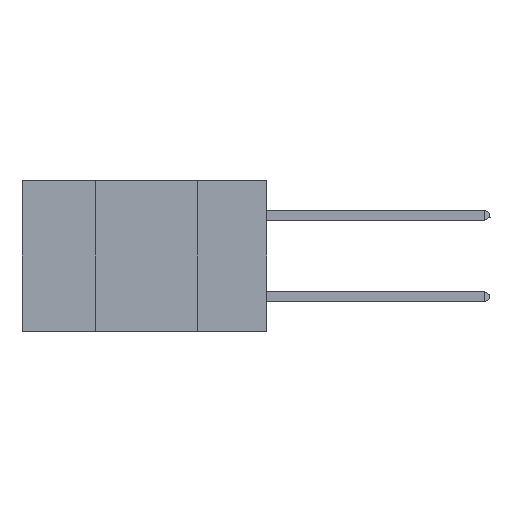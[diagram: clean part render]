
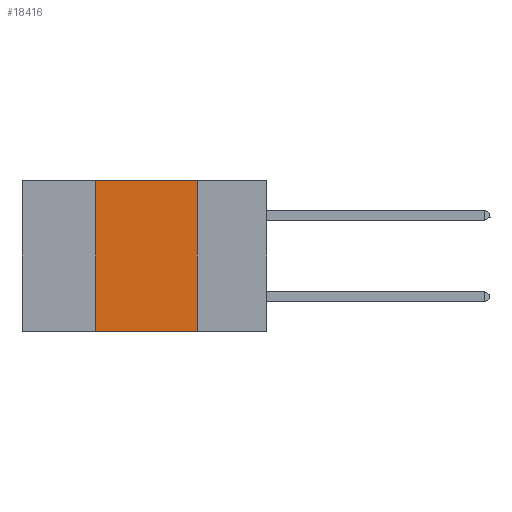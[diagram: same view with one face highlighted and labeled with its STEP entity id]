
A CAD part, left-side view. The second image highlights one B-rep face of the part: STEP entity #18416.
In plain terms, the highlighted planar face has unit normal (-1, 0, 0).
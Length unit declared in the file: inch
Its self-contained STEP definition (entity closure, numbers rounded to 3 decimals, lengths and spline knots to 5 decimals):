
#700 = CARTESIAN_POINT ( 'NONE',  ( 0., 0.42, -0.37 ) ) ;
#1457 = ORIENTED_EDGE ( 'NONE', *, *, #24582, .F. ) ;
#3291 = VERTEX_POINT ( 'NONE', #20561 ) ;
#4500 = LINE ( 'NONE', #32602, #20239 ) ;
#4933 = ORIENTED_EDGE ( 'NONE', *, *, #39990, .F. ) ;
#5363 = EDGE_CURVE ( 'NONE', #10061, #11072, #24682, .T. ) ;
#6220 = ORIENTED_EDGE ( 'NONE', *, *, #5363, .F. ) ;
#8501 = FACE_OUTER_BOUND ( 'NONE', #34142, .T. ) ;
#8634 = DIRECTION ( 'NONE',  ( 0., -1., 0. ) ) ;
#10061 = VERTEX_POINT ( 'NONE', #700 ) ;
#10278 = DIRECTION ( 'NONE',  ( 0., 0., 1. ) ) ;
#11072 = VERTEX_POINT ( 'NONE', #42712 ) ;
#11085 = PLANE ( 'NONE',  #21429 ) ;
#12824 = VECTOR ( 'NONE', #10278, 39.37008 ) ;
#15388 = LINE ( 'NONE', #29550, #35686 ) ;
#18416 = ADVANCED_FACE ( 'NONE', ( #8501 ), #11085, .F. ) ;
#20239 = VECTOR ( 'NONE', #45882, 39.37008 ) ;
#20561 = CARTESIAN_POINT ( 'NONE',  ( 0., 0.17, -0.37 ) ) ;
#21429 = AXIS2_PLACEMENT_3D ( 'NONE', #29192, #39649, #32898 ) ;
#21644 = CARTESIAN_POINT ( 'NONE',  ( 0., 0.42, 0. ) ) ;
#24582 = EDGE_CURVE ( 'NONE', #40576, #3291, #4500, .T. ) ;
#24682 = LINE ( 'NONE', #21644, #12824 ) ;
#25158 = DIRECTION ( 'NONE',  ( 0., -1., 0. ) ) ;
#29192 = CARTESIAN_POINT ( 'NONE',  ( 0., 0.6, 0. ) ) ;
#29242 = VECTOR ( 'NONE', #8634, 39.37008 ) ;
#29550 = CARTESIAN_POINT ( 'NONE',  ( 0., 0.6, -0.37 ) ) ;
#32602 = CARTESIAN_POINT ( 'NONE',  ( 0., 0.17, 0. ) ) ;
#32898 = DIRECTION ( 'NONE',  ( 0., 0., -1. ) ) ;
#33898 = CARTESIAN_POINT ( 'NONE',  ( 0., 0.17, 0. ) ) ;
#34142 = EDGE_LOOP ( 'NONE', ( #1457, #4933, #6220, #39205 ) ) ;
#35686 = VECTOR ( 'NONE', #25158, 39.37008 ) ;
#36899 = EDGE_CURVE ( 'NONE', #10061, #3291, #15388, .T. ) ;
#39205 = ORIENTED_EDGE ( 'NONE', *, *, #36899, .T. ) ;
#39649 = DIRECTION ( 'NONE',  ( 1., 0., 0. ) ) ;
#39990 = EDGE_CURVE ( 'NONE', #11072, #40576, #43502, .T. ) ;
#40238 = CARTESIAN_POINT ( 'NONE',  ( 0., 0.6, 0. ) ) ;
#40576 = VERTEX_POINT ( 'NONE', #33898 ) ;
#42712 = CARTESIAN_POINT ( 'NONE',  ( 0., 0.42, 0. ) ) ;
#43502 = LINE ( 'NONE', #40238, #29242 ) ;
#45882 = DIRECTION ( 'NONE',  ( 0., 0., -1. ) ) ;
